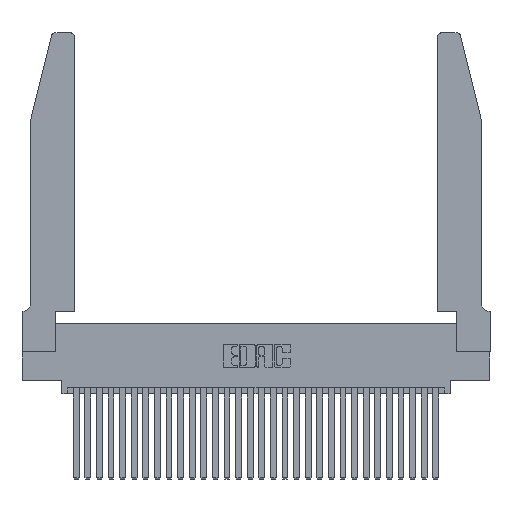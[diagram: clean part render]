
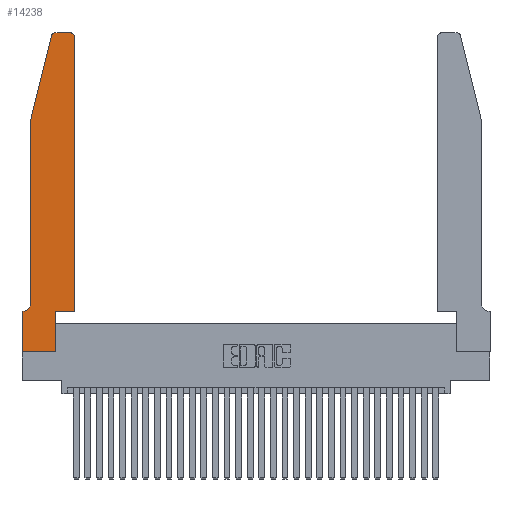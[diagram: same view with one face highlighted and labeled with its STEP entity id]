
A CAD part, top view. The second image highlights one B-rep face of the part: STEP entity #14238.
In plain terms, the highlighted planar face has unit normal (0, 0, 1).
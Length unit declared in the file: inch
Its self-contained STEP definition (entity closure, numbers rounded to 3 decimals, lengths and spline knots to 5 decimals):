
#408 = CARTESIAN_POINT ( 'NONE',  ( 0.2865, 0.35, 0.37 ) ) ;
#494 = EDGE_CURVE ( 'NONE', #4680, #21464, #19147, .T. ) ;
#952 = DIRECTION ( 'NONE',  ( 0., 0., 1. ) ) ;
#1604 = DIRECTION ( 'NONE',  ( 0., 1., 0. ) ) ;
#2111 = VERTEX_POINT ( 'NONE', #15411 ) ;
#2159 = ORIENTED_EDGE ( 'NONE', *, *, #2584, .T. ) ;
#2584 = EDGE_CURVE ( 'NONE', #21464, #27791, #5480, .T. ) ;
#2907 = DIRECTION ( 'NONE',  ( 0., 1., 0. ) ) ;
#2983 = EDGE_LOOP ( 'NONE', ( #6792, #13933, #26559, #10541, #24691, #12810, #7930, #2159, #29206, #12466, #25081, #8313 ) ) ;
#3448 = EDGE_CURVE ( 'NONE', #27791, #4972, #13034, .T. ) ;
#3568 = CARTESIAN_POINT ( 'NONE',  ( 0.0755, 2., 0.37 ) ) ;
#3806 = EDGE_CURVE ( 'NONE', #6044, #18769, #29401, .T. ) ;
#4007 = DIRECTION ( 'NONE',  ( 0., 0., 1. ) ) ;
#4680 = VERTEX_POINT ( 'NONE', #16811 ) ;
#4972 = VERTEX_POINT ( 'NONE', #20095 ) ;
#5480 = LINE ( 'NONE', #25421, #29417 ) ;
#5563 = CIRCLE ( 'NONE', #28305, 0.07 ) ;
#6044 = VERTEX_POINT ( 'NONE', #22266 ) ;
#6557 = DIRECTION ( 'NONE',  ( -0.239, -0.971, 0. ) ) ;
#6772 = CARTESIAN_POINT ( 'NONE',  ( 0.4505, 0.35, 0.37 ) ) ;
#6792 = ORIENTED_EDGE ( 'NONE', *, *, #20984, .T. ) ;
#6927 = AXIS2_PLACEMENT_3D ( 'NONE', #18409, #4007, #20795 ) ;
#7287 = FACE_OUTER_BOUND ( 'NONE', #2983, .T. ) ;
#7351 = VECTOR ( 'NONE', #30454, 39.37008 ) ;
#7624 = CARTESIAN_POINT ( 'NONE',  ( 0.0055, 0.42, 0.37 ) ) ;
#7930 = ORIENTED_EDGE ( 'NONE', *, *, #494, .T. ) ;
#8313 = ORIENTED_EDGE ( 'NONE', *, *, #13951, .T. ) ;
#8622 = LINE ( 'NONE', #16526, #19834 ) ;
#9020 = DIRECTION ( 'NONE',  ( 0., -1., 0. ) ) ;
#9050 = CARTESIAN_POINT ( 'NONE',  ( 0., 0., 0.37 ) ) ;
#9155 = VERTEX_POINT ( 'NONE', #3568 ) ;
#9313 = EDGE_CURVE ( 'NONE', #26120, #10399, #31086, .T. ) ;
#9362 = DIRECTION ( 'NONE',  ( 0., 0., 1. ) ) ;
#10031 = DIRECTION ( 'NONE',  ( -1., 0., 0. ) ) ;
#10399 = VERTEX_POINT ( 'NONE', #24875 ) ;
#10541 = ORIENTED_EDGE ( 'NONE', *, *, #12079, .T. ) ;
#12079 = EDGE_CURVE ( 'NONE', #9155, #16812, #22704, .T. ) ;
#12466 = ORIENTED_EDGE ( 'NONE', *, *, #20721, .T. ) ;
#12810 = ORIENTED_EDGE ( 'NONE', *, *, #17297, .T. ) ;
#13034 = LINE ( 'NONE', #408, #24918 ) ;
#13114 = PLANE ( 'NONE',  #14503 ) ;
#13225 = VERTEX_POINT ( 'NONE', #23160 ) ;
#13598 = DIRECTION ( 'NONE',  ( 1., 0., 0. ) ) ;
#13726 = LINE ( 'NONE', #6772, #7351 ) ;
#13820 = CARTESIAN_POINT ( 'NONE',  ( 0.0755, 2., 0.37 ) ) ;
#13933 = ORIENTED_EDGE ( 'NONE', *, *, #3806, .T. ) ;
#13951 = EDGE_CURVE ( 'NONE', #10399, #13225, #28185, .T. ) ;
#14238 = ADVANCED_FACE ( 'NONE', ( #7287 ), #13114, .T. ) ;
#14503 = AXIS2_PLACEMENT_3D ( 'NONE', #29761, #952, #17887 ) ;
#15026 = DIRECTION ( 'NONE',  ( -1., 0., 0. ) ) ;
#15411 = CARTESIAN_POINT ( 'NONE',  ( 0.0055, 0.35, 0.37 ) ) ;
#15773 = VECTOR ( 'NONE', #6557, 39.37008 ) ;
#16122 = CARTESIAN_POINT ( 'NONE',  ( 0.4505, 0.35, 0.37 ) ) ;
#16526 = CARTESIAN_POINT ( 'NONE',  ( 0.0755, 0.35, 0.37 ) ) ;
#16533 = LINE ( 'NONE', #13820, #15773 ) ;
#16739 = EDGE_CURVE ( 'NONE', #18769, #9155, #16533, .T. ) ;
#16811 = CARTESIAN_POINT ( 'NONE',  ( 0., 0.35, 0.37 ) ) ;
#16812 = VERTEX_POINT ( 'NONE', #28366 ) ;
#16888 = CARTESIAN_POINT ( 'NONE',  ( 0., 0., 0.37 ) ) ;
#17297 = EDGE_CURVE ( 'NONE', #2111, #4680, #8622, .T. ) ;
#17444 = EDGE_CURVE ( 'NONE', #16812, #2111, #5563, .T. ) ;
#17887 = DIRECTION ( 'NONE',  ( 1., 0., 0. ) ) ;
#18150 = LINE ( 'NONE', #26867, #30825 ) ;
#18273 = AXIS2_PLACEMENT_3D ( 'NONE', #23628, #9362, #26034 ) ;
#18409 = CARTESIAN_POINT ( 'NONE',  ( 0.284, 2.72, 0.37 ) ) ;
#18769 = VERTEX_POINT ( 'NONE', #29965 ) ;
#19147 = LINE ( 'NONE', #9050, #24680 ) ;
#19834 = VECTOR ( 'NONE', #23690, 39.37008 ) ;
#20095 = CARTESIAN_POINT ( 'NONE',  ( 0.2865, 0.35, 0.37 ) ) ;
#20721 = EDGE_CURVE ( 'NONE', #4972, #26120, #13726, .T. ) ;
#20795 = DIRECTION ( 'NONE',  ( 1., 0., 0. ) ) ;
#20984 = EDGE_CURVE ( 'NONE', #13225, #6044, #18150, .T. ) ;
#21244 = CARTESIAN_POINT ( 'NONE',  ( 0.0755, 2., 0.37 ) ) ;
#21464 = VERTEX_POINT ( 'NONE', #16888 ) ;
#21948 = VECTOR ( 'NONE', #23636, 39.37008 ) ;
#22266 = CARTESIAN_POINT ( 'NONE',  ( 0.284, 2.75, 0.37 ) ) ;
#22704 = LINE ( 'NONE', #21244, #21948 ) ;
#23160 = CARTESIAN_POINT ( 'NONE',  ( 0.4205, 2.75, 0.37 ) ) ;
#23628 = CARTESIAN_POINT ( 'NONE',  ( 0.4205, 2.72, 0.37 ) ) ;
#23636 = DIRECTION ( 'NONE',  ( 0., -1., 0. ) ) ;
#23690 = DIRECTION ( 'NONE',  ( -1., 0., 0. ) ) ;
#24278 = DIRECTION ( 'NONE',  ( 0., 0., -1. ) ) ;
#24680 = VECTOR ( 'NONE', #9020, 39.37008 ) ;
#24691 = ORIENTED_EDGE ( 'NONE', *, *, #17444, .T. ) ;
#24721 = VECTOR ( 'NONE', #1604, 39.37008 ) ;
#24875 = CARTESIAN_POINT ( 'NONE',  ( 0.4505, 2.72, 0.37 ) ) ;
#24918 = VECTOR ( 'NONE', #2907, 39.37008 ) ;
#25081 = ORIENTED_EDGE ( 'NONE', *, *, #9313, .T. ) ;
#25421 = CARTESIAN_POINT ( 'NONE',  ( 0., 0., 0.37 ) ) ;
#26034 = DIRECTION ( 'NONE',  ( 1., 0., 0. ) ) ;
#26120 = VERTEX_POINT ( 'NONE', #30754 ) ;
#26559 = ORIENTED_EDGE ( 'NONE', *, *, #16739, .T. ) ;
#26867 = CARTESIAN_POINT ( 'NONE',  ( 0.2605, 2.75, 0.37 ) ) ;
#27791 = VERTEX_POINT ( 'NONE', #30656 ) ;
#28185 = CIRCLE ( 'NONE', #18273, 0.03 ) ;
#28305 = AXIS2_PLACEMENT_3D ( 'NONE', #7624, #24278, #10031 ) ;
#28366 = CARTESIAN_POINT ( 'NONE',  ( 0.0755, 0.42, 0.37 ) ) ;
#29206 = ORIENTED_EDGE ( 'NONE', *, *, #3448, .T. ) ;
#29401 = CIRCLE ( 'NONE', #6927, 0.03 ) ;
#29417 = VECTOR ( 'NONE', #13598, 39.37008 ) ;
#29761 = CARTESIAN_POINT ( 'NONE',  ( 0., 0.35, 0.37 ) ) ;
#29965 = CARTESIAN_POINT ( 'NONE',  ( 0.25487, 2.72718, 0.37 ) ) ;
#30454 = DIRECTION ( 'NONE',  ( 1., 0., 0. ) ) ;
#30656 = CARTESIAN_POINT ( 'NONE',  ( 0.2865, 0., 0.37 ) ) ;
#30754 = CARTESIAN_POINT ( 'NONE',  ( 0.4505, 0.35, 0.37 ) ) ;
#30825 = VECTOR ( 'NONE', #15026, 39.37008 ) ;
#31086 = LINE ( 'NONE', #16122, #24721 ) ;
